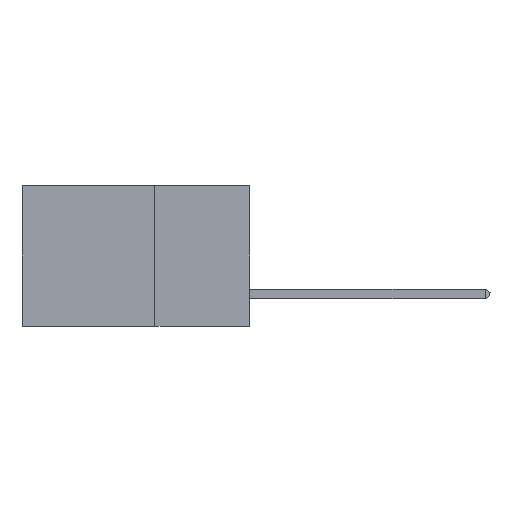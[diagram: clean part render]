
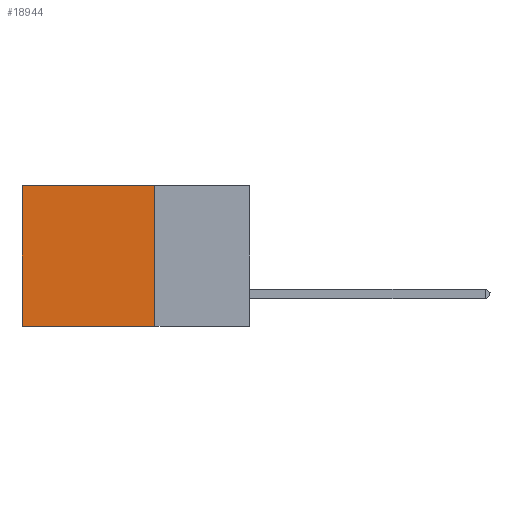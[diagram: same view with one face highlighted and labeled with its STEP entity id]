
A CAD part, left-side view. The second image highlights one B-rep face of the part: STEP entity #18944.
In plain terms, the highlighted planar face has unit normal (-1, 0, 0).
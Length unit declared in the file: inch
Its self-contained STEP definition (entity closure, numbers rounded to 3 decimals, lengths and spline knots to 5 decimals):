
#63 = VERTEX_POINT ( 'NONE', #14835 ) ;
#634 = LINE ( 'NONE', #15097, #19324 ) ;
#1398 = VECTOR ( 'NONE', #16314, 39.37008 ) ;
#2717 = DIRECTION ( 'NONE',  ( 0., 0., -1. ) ) ;
#5460 = CARTESIAN_POINT ( 'NONE',  ( 0.2875, 0.25, 0. ) ) ;
#8298 = VERTEX_POINT ( 'NONE', #5460 ) ;
#8663 = CARTESIAN_POINT ( 'NONE',  ( 0.2875, 0.25, 0. ) ) ;
#9144 = CARTESIAN_POINT ( 'NONE',  ( 0.2875, 0.25, 0. ) ) ;
#9814 = ORIENTED_EDGE ( 'NONE', *, *, #18367, .T. ) ;
#9822 = AXIS2_PLACEMENT_3D ( 'NONE', #18911, #11546, #2717 ) ;
#10576 = EDGE_LOOP ( 'NONE', ( #9814, #20534, #26844, #13296 ) ) ;
#10670 = CARTESIAN_POINT ( 'NONE',  ( 0.2875, 0.6, -0.37 ) ) ;
#10802 = VECTOR ( 'NONE', #11636, 39.37008 ) ;
#11546 = DIRECTION ( 'NONE',  ( 1., 0., 0. ) ) ;
#11636 = DIRECTION ( 'NONE',  ( 0., 1., 0. ) ) ;
#12002 = LINE ( 'NONE', #9144, #10802 ) ;
#13296 = ORIENTED_EDGE ( 'NONE', *, *, #17104, .T. ) ;
#13580 = CARTESIAN_POINT ( 'NONE',  ( 0.2875, 0.6, 0. ) ) ;
#13947 = PLANE ( 'NONE',  #9822 ) ;
#14835 = CARTESIAN_POINT ( 'NONE',  ( 0.2875, 0.25, -0.37 ) ) ;
#15097 = CARTESIAN_POINT ( 'NONE',  ( 0.2875, 0.6, 0. ) ) ;
#16314 = DIRECTION ( 'NONE',  ( 0., 1., 0. ) ) ;
#17104 = EDGE_CURVE ( 'NONE', #8298, #19662, #12002, .T. ) ;
#18367 = EDGE_CURVE ( 'NONE', #19662, #20597, #634, .T. ) ;
#18911 = CARTESIAN_POINT ( 'NONE',  ( 0.2875, 0.25, 0. ) ) ;
#18944 = ADVANCED_FACE ( 'NONE', ( #30576 ), #13947, .F. ) ;
#19324 = VECTOR ( 'NONE', #20099, 39.37008 ) ;
#19662 = VERTEX_POINT ( 'NONE', #13580 ) ;
#20099 = DIRECTION ( 'NONE',  ( 0., 0., -1. ) ) ;
#20534 = ORIENTED_EDGE ( 'NONE', *, *, #31378, .F. ) ;
#20597 = VERTEX_POINT ( 'NONE', #10670 ) ;
#20986 = LINE ( 'NONE', #8663, #22148 ) ;
#22148 = VECTOR ( 'NONE', #23754, 39.37008 ) ;
#23754 = DIRECTION ( 'NONE',  ( 0., 0., -1. ) ) ;
#26698 = LINE ( 'NONE', #30897, #1398 ) ;
#26844 = ORIENTED_EDGE ( 'NONE', *, *, #29012, .F. ) ;
#29012 = EDGE_CURVE ( 'NONE', #8298, #63, #20986, .T. ) ;
#30576 = FACE_OUTER_BOUND ( 'NONE', #10576, .T. ) ;
#30897 = CARTESIAN_POINT ( 'NONE',  ( 0.2875, 0.25, -0.37 ) ) ;
#31378 = EDGE_CURVE ( 'NONE', #63, #20597, #26698, .T. ) ;
